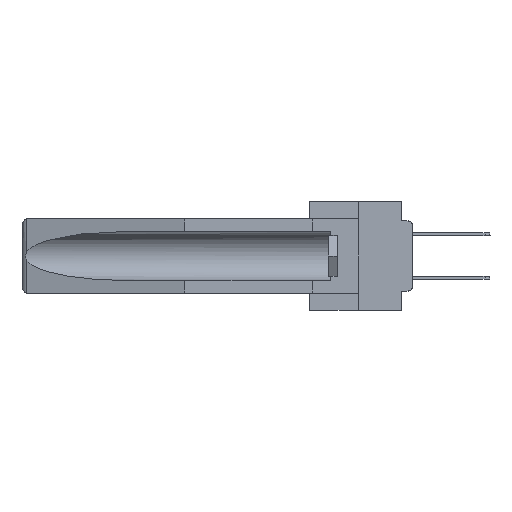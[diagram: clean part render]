
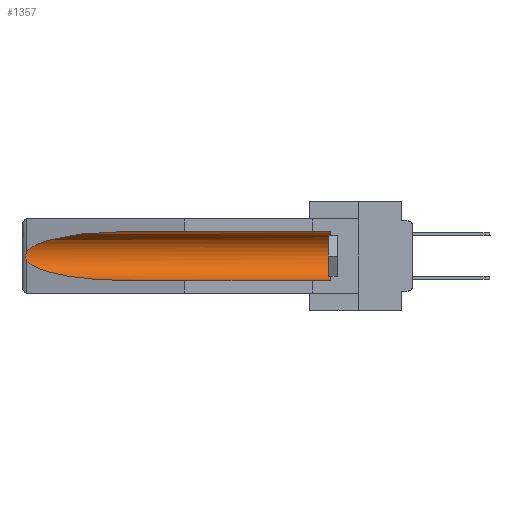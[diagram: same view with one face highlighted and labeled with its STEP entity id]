
A CAD part, left-side view. The second image highlights one B-rep face of the part: STEP entity #1357.
In plain terms, the highlighted cylindrical face has radius 2.857 mm (diameter 5.715 mm), a partial arc.
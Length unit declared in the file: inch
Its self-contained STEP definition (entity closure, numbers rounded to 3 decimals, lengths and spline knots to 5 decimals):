
#454 = ORIENTED_EDGE ( 'NONE', *, *, #20787, .T. ) ;
#732 = CARTESIAN_POINT ( 'NONE',  ( 0.155, -0.30754, -0.284 ) ) ;
#875 = CARTESIAN_POINT ( 'NONE',  ( 0.26537, 1.52718, -0.19328 ) ) ;
#1357 = ADVANCED_FACE ( 'NONE', ( #1666 ), #20686, .F. ) ;
#1666 = FACE_OUTER_BOUND ( 'NONE', #30590, .T. ) ;
#2145 = AXIS2_PLACEMENT_3D ( 'NONE', #19300, #24254, #26744 ) ;
#2497 = DIRECTION ( 'NONE',  ( 0., 0., 1. ) ) ;
#2533 = CARTESIAN_POINT ( 'NONE',  ( 0.26654, 1.53092, -0.15636 ) ) ;
#2730 = CARTESIAN_POINT ( 'NONE',  ( 0.2675, 1.53308, -0.17534 ) ) ;
#4208 = CARTESIAN_POINT ( 'NONE',  ( 0.25451, 1.48313, -0.24835 ) ) ;
#4228 = EDGE_CURVE ( 'NONE', #4591, #28480, #29774, .T. ) ;
#4591 = VERTEX_POINT ( 'NONE', #875 ) ;
#4900 = ORIENTED_EDGE ( 'NONE', *, *, #25256, .T. ) ;
#5166 = CARTESIAN_POINT ( 'NONE',  ( 0.26537, 1.52718, -0.19328 ) ) ;
#6147 = B_SPLINE_CURVE_WITH_KNOTS ( 'NONE', 3,
 ( #9242, #24193, #2533, #10206, #19884, #2730, #15013, #9992, #29066, #12598 ),
 .UNSPECIFIED., .F., .F.,
 ( 4, 2, 2, 2, 4 ),
 ( 0., 0.00029, 0.00058, 0.00087, 0.00117 ),
 .UNSPECIFIED. ) ;
#6663 = CARTESIAN_POINT ( 'NONE',  ( 0.155, 1.07973, -0.284 ) ) ;
#7299 = CARTESIAN_POINT ( 'NONE',  ( 0.21114, 1.30732, -0.059 ) ) ;
#7437 = CARTESIAN_POINT ( 'NONE',  ( 0.155, 1.07973, -0.284 ) ) ;
#9242 = CARTESIAN_POINT ( 'NONE',  ( 0.26537, 1.52718, -0.14972 ) ) ;
#9369 = EDGE_CURVE ( 'NONE', #11519, #28480, #24280, .T. ) ;
#9608 = CIRCLE ( 'NONE', #26326, 0.1125 ) ;
#9992 = CARTESIAN_POINT ( 'NONE',  ( 0.26655, 1.53094, -0.18657 ) ) ;
#10206 = CARTESIAN_POINT ( 'NONE',  ( 0.2673, 1.5327, -0.16383 ) ) ;
#11519 = VERTEX_POINT ( 'NONE', #13906 ) ;
#12598 = CARTESIAN_POINT ( 'NONE',  ( 0.26537, 1.52718, -0.19328 ) ) ;
#13820 = EDGE_CURVE ( 'NONE', #24378, #18281, #16290, .T. ) ;
#13906 = CARTESIAN_POINT ( 'NONE',  ( 0.155, 0.126, -0.284 ) ) ;
#14631 = CARTESIAN_POINT ( 'NONE',  ( 0.21114, 1.30732, -0.284 ) ) ;
#14800 = EDGE_CURVE ( 'NONE', #16481, #24378, #29315, .T. ) ;
#15013 = CARTESIAN_POINT ( 'NONE',  ( 0.2673, 1.53269, -0.17917 ) ) ;
#15256 = ORIENTED_EDGE ( 'NONE', *, *, #14800, .T. ) ;
#15295 = CARTESIAN_POINT ( 'NONE',  ( 0.155, -0.30754, -0.059 ) ) ;
#16290 =( BOUNDED_CURVE ( )  B_SPLINE_CURVE ( 3, ( #22178, #7299, #26810, #24316 ),
 .UNSPECIFIED., .F., .F. ) 
 B_SPLINE_CURVE_WITH_KNOTS ( ( 4, 4 ),
 ( 4.71239, 6.08839 ),
 .UNSPECIFIED. ) 
 CURVE ( )  GEOMETRIC_REPRESENTATION_ITEM ( )  RATIONAL_B_SPLINE_CURVE ( ( 1., 0.848, 0.848, 1. ) ) 
 REPRESENTATION_ITEM ( '' )  );
#16481 = VERTEX_POINT ( 'NONE', #31460 ) ;
#18281 = VERTEX_POINT ( 'NONE', #30905 ) ;
#18480 = VECTOR ( 'NONE', #27617, 39.37008 ) ;
#18957 = CARTESIAN_POINT ( 'NONE',  ( 0.155, 1.07973, -0.059 ) ) ;
#19300 = CARTESIAN_POINT ( 'NONE',  ( 0.155, -0.30754, -0.1715 ) ) ;
#19340 = ORIENTED_EDGE ( 'NONE', *, *, #4228, .T. ) ;
#19884 = CARTESIAN_POINT ( 'NONE',  ( 0.2675, 1.53308, -0.16763 ) ) ;
#20686 = CYLINDRICAL_SURFACE ( 'NONE', #2145, 0.1125 ) ;
#20787 = EDGE_CURVE ( 'NONE', #11519, #16481, #9608, .T. ) ;
#22178 = CARTESIAN_POINT ( 'NONE',  ( 0.155, 1.07973, -0.059 ) ) ;
#22651 = DIRECTION ( 'NONE',  ( 0., -1., 0. ) ) ;
#23611 = ORIENTED_EDGE ( 'NONE', *, *, #13820, .T. ) ;
#24193 = CARTESIAN_POINT ( 'NONE',  ( 0.26597, 1.52961, -0.15275 ) ) ;
#24254 = DIRECTION ( 'NONE',  ( 0., 1., 0. ) ) ;
#24280 = LINE ( 'NONE', #732, #29710 ) ;
#24316 = CARTESIAN_POINT ( 'NONE',  ( 0.26537, 1.52718, -0.14972 ) ) ;
#24378 = VERTEX_POINT ( 'NONE', #18957 ) ;
#24999 = DIRECTION ( 'NONE',  ( 0., 1., 0. ) ) ;
#25256 = EDGE_CURVE ( 'NONE', #18281, #4591, #6147, .T. ) ;
#26326 = AXIS2_PLACEMENT_3D ( 'NONE', #27397, #22651, #2497 ) ;
#26744 = DIRECTION ( 'NONE',  ( 0., 0., 1. ) ) ;
#26810 = CARTESIAN_POINT ( 'NONE',  ( 0.25451, 1.48313, -0.09465 ) ) ;
#27397 = CARTESIAN_POINT ( 'NONE',  ( 0.155, 0.126, -0.1715 ) ) ;
#27617 = DIRECTION ( 'NONE',  ( 0., 1., 0. ) ) ;
#28119 = ORIENTED_EDGE ( 'NONE', *, *, #9369, .F. ) ;
#28480 = VERTEX_POINT ( 'NONE', #6663 ) ;
#29066 = CARTESIAN_POINT ( 'NONE',  ( 0.26597, 1.5296, -0.19026 ) ) ;
#29315 = LINE ( 'NONE', #15295, #18480 ) ;
#29710 = VECTOR ( 'NONE', #24999, 39.37008 ) ;
#29774 =( BOUNDED_CURVE ( )  B_SPLINE_CURVE ( 3, ( #5166, #4208, #14631, #7437 ),
 .UNSPECIFIED., .F., .F. ) 
 B_SPLINE_CURVE_WITH_KNOTS ( ( 4, 4 ),
 ( 0.1948, 1.5708 ),
 .UNSPECIFIED. ) 
 CURVE ( )  GEOMETRIC_REPRESENTATION_ITEM ( )  RATIONAL_B_SPLINE_CURVE ( ( 1., 0.848, 0.848, 1. ) ) 
 REPRESENTATION_ITEM ( '' )  );
#30590 = EDGE_LOOP ( 'NONE', ( #23611, #4900, #19340, #28119, #454, #15256 ) ) ;
#30905 = CARTESIAN_POINT ( 'NONE',  ( 0.26537, 1.52718, -0.14972 ) ) ;
#31460 = CARTESIAN_POINT ( 'NONE',  ( 0.155, 0.126, -0.059 ) ) ;
